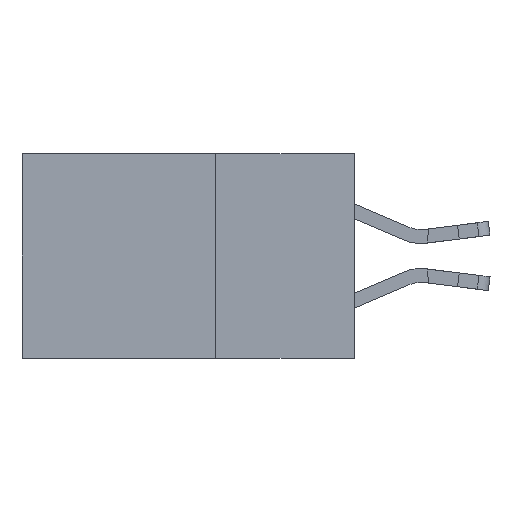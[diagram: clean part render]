
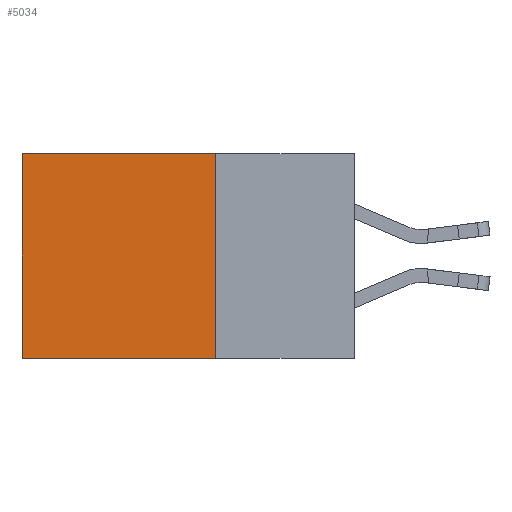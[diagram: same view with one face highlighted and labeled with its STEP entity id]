
A CAD part, left-side view. The second image highlights one B-rep face of the part: STEP entity #5034.
In plain terms, the highlighted planar face has unit normal (-1, 0, 0).
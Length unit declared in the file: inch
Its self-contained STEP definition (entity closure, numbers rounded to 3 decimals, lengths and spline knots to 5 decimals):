
#781 = CARTESIAN_POINT ( 'NONE',  ( 0.298, 0.6, -0.37 ) ) ;
#1237 = CARTESIAN_POINT ( 'NONE',  ( 0.298, 0.25, 0. ) ) ;
#2037 = VERTEX_POINT ( 'NONE', #1237 ) ;
#2181 = CARTESIAN_POINT ( 'NONE',  ( 0.298, 0.6, 0. ) ) ;
#2261 = CARTESIAN_POINT ( 'NONE',  ( 0.298, 0.25, 0. ) ) ;
#2867 = EDGE_CURVE ( 'NONE', #2037, #4028, #11111, .T. ) ;
#3188 = CARTESIAN_POINT ( 'NONE',  ( 0.298, 0.25, 0. ) ) ;
#3291 = VECTOR ( 'NONE', #5091, 39.37008 ) ;
#3719 = DIRECTION ( 'NONE',  ( 0., 0., -1. ) ) ;
#4028 = VERTEX_POINT ( 'NONE', #10401 ) ;
#5034 = ADVANCED_FACE ( 'NONE', ( #11103 ), #7603, .F. ) ;
#5091 = DIRECTION ( 'NONE',  ( 0., 0., -1. ) ) ;
#5796 = VECTOR ( 'NONE', #12473, 39.37008 ) ;
#6141 = ORIENTED_EDGE ( 'NONE', *, *, #10368, .F. ) ;
#6598 = LINE ( 'NONE', #15250, #7243 ) ;
#6859 = LINE ( 'NONE', #9614, #5796 ) ;
#7243 = VECTOR ( 'NONE', #16698, 39.37008 ) ;
#7335 = VERTEX_POINT ( 'NONE', #781 ) ;
#7452 = DIRECTION ( 'NONE',  ( 0., 0., -1. ) ) ;
#7603 = PLANE ( 'NONE',  #7676 ) ;
#7676 = AXIS2_PLACEMENT_3D ( 'NONE', #2261, #9001, #3719 ) ;
#7869 = ORIENTED_EDGE ( 'NONE', *, *, #2867, .F. ) ;
#9001 = DIRECTION ( 'NONE',  ( 1., 0., 0. ) ) ;
#9113 = VECTOR ( 'NONE', #7452, 39.37008 ) ;
#9614 = CARTESIAN_POINT ( 'NONE',  ( 0.298, 0.25, -0.37 ) ) ;
#10368 = EDGE_CURVE ( 'NONE', #4028, #7335, #6859, .T. ) ;
#10401 = CARTESIAN_POINT ( 'NONE',  ( 0.298, 0.25, -0.37 ) ) ;
#11103 = FACE_OUTER_BOUND ( 'NONE', #14064, .T. ) ;
#11111 = LINE ( 'NONE', #3188, #9113 ) ;
#12473 = DIRECTION ( 'NONE',  ( 0., 1., 0. ) ) ;
#13056 = EDGE_CURVE ( 'NONE', #2037, #13842, #6598, .T. ) ;
#13373 = ORIENTED_EDGE ( 'NONE', *, *, #13056, .T. ) ;
#13481 = LINE ( 'NONE', #17444, #3291 ) ;
#13842 = VERTEX_POINT ( 'NONE', #2181 ) ;
#14064 = EDGE_LOOP ( 'NONE', ( #15545, #6141, #7869, #13373 ) ) ;
#15250 = CARTESIAN_POINT ( 'NONE',  ( 0.298, 0.25, 0. ) ) ;
#15265 = EDGE_CURVE ( 'NONE', #13842, #7335, #13481, .T. ) ;
#15545 = ORIENTED_EDGE ( 'NONE', *, *, #15265, .T. ) ;
#16698 = DIRECTION ( 'NONE',  ( 0., 1., 0. ) ) ;
#17444 = CARTESIAN_POINT ( 'NONE',  ( 0.298, 0.6, 0. ) ) ;
